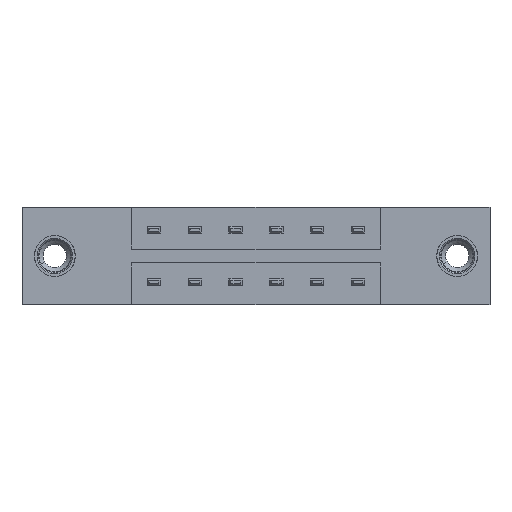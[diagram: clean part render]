
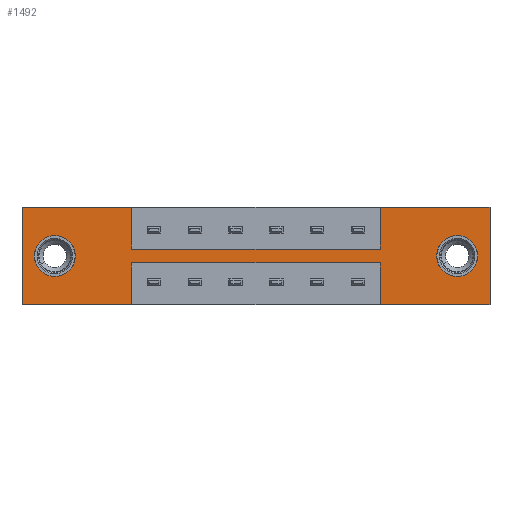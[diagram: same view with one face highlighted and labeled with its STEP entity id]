
A CAD part, front view. The second image highlights one B-rep face of the part: STEP entity #1492.
In plain terms, the highlighted planar face has unit normal (0, -1, 0).
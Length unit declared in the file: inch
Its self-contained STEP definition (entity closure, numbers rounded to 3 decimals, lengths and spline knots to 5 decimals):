
#13 = ORIENTED_EDGE ( 'NONE', *, *, #5651, .T. ) ;
#305 = ORIENTED_EDGE ( 'NONE', *, *, #8536, .F. ) ;
#362 = AXIS2_PLACEMENT_3D ( 'NONE', #4719, #4704, #4684 ) ;
#561 = VECTOR ( 'NONE', #1342, 39.37008 ) ;
#596 = DIRECTION ( 'NONE',  ( 0., 0., 1. ) ) ;
#611 = DIRECTION ( 'NONE',  ( 0., 1., 0. ) ) ;
#632 = CARTESIAN_POINT ( 'NONE',  ( 0.125, 0., -0.185 ) ) ;
#669 = ORIENTED_EDGE ( 'NONE', *, *, #1375, .T. ) ;
#816 = VERTEX_POINT ( 'NONE', #7714 ) ;
#878 = LINE ( 'NONE', #2511, #6748 ) ;
#913 = EDGE_CURVE ( 'NONE', #7745, #5572, #878, .T. ) ;
#1073 = VECTOR ( 'NONE', #7024, 39.37008 ) ;
#1323 = EDGE_CURVE ( 'NONE', #5572, #7181, #4646, .T. ) ;
#1342 = DIRECTION ( 'NONE',  ( 0., 0., 1. ) ) ;
#1375 = EDGE_CURVE ( 'NONE', #6483, #5742, #3723, .T. ) ;
#1381 = EDGE_LOOP ( 'NONE', ( #4957, #2207, #7634, #305, #5319, #8008, #8800, #1449, #4160, #9099, #5473, #8551 ) ) ;
#1449 = ORIENTED_EDGE ( 'NONE', *, *, #7810, .F. ) ;
#1492 = ADVANCED_FACE ( 'NONE', ( #7699, #2367, #5896 ), #2738, .T. ) ;
#1685 = CARTESIAN_POINT ( 'NONE',  ( 1.784, 0., 0. ) ) ;
#1892 = CARTESIAN_POINT ( 'NONE',  ( 1.3665, 0., -0.1585 ) ) ;
#1949 = VERTEX_POINT ( 'NONE', #8513 ) ;
#2194 = VERTEX_POINT ( 'NONE', #6733 ) ;
#2195 = LINE ( 'NONE', #5640, #9402 ) ;
#2207 = ORIENTED_EDGE ( 'NONE', *, *, #913, .F. ) ;
#2288 = VERTEX_POINT ( 'NONE', #5562 ) ;
#2299 = LINE ( 'NONE', #7814, #5845 ) ;
#2314 = LINE ( 'NONE', #1685, #7653 ) ;
#2346 = DIRECTION ( 'NONE',  ( -1., 0., 0. ) ) ;
#2367 = FACE_BOUND ( 'NONE', #9194, .T. ) ;
#2501 = VECTOR ( 'NONE', #6003, 39.37008 ) ;
#2511 = CARTESIAN_POINT ( 'NONE',  ( 0., 0., -0.37 ) ) ;
#2539 = LINE ( 'NONE', #6915, #6027 ) ;
#2600 = EDGE_CURVE ( 'NONE', #2288, #8261, #2843, .T. ) ;
#2736 = DIRECTION ( 'NONE',  ( 0., 0., -1. ) ) ;
#2738 = PLANE ( 'NONE',  #8091 ) ;
#2800 = CARTESIAN_POINT ( 'NONE',  ( 0.125, 0., -0.107 ) ) ;
#2802 = CARTESIAN_POINT ( 'NONE',  ( 0., 0., -0.37 ) ) ;
#2821 = LINE ( 'NONE', #5255, #8122 ) ;
#2832 = DIRECTION ( 'NONE',  ( 0., -1., 0. ) ) ;
#2843 = LINE ( 'NONE', #1892, #561 ) ;
#3033 = EDGE_CURVE ( 'NONE', #4695, #816, #2539, .T. ) ;
#3245 = DIRECTION ( 'NONE',  ( 0., 0., -1. ) ) ;
#3529 = CIRCLE ( 'NONE', #9371, 0.078 ) ;
#3587 = CARTESIAN_POINT ( 'NONE',  ( 1.659, 0., -0.185 ) ) ;
#3657 = VERTEX_POINT ( 'NONE', #8221 ) ;
#3663 = CARTESIAN_POINT ( 'NONE',  ( 0., 0., 0. ) ) ;
#3723 = CIRCLE ( 'NONE', #362, 0.078 ) ;
#3750 = ORIENTED_EDGE ( 'NONE', *, *, #4228, .T. ) ;
#3890 = AXIS2_PLACEMENT_3D ( 'NONE', #8607, #4503, #9289 ) ;
#3987 = CARTESIAN_POINT ( 'NONE',  ( 1.784, 0., -0.37 ) ) ;
#4000 = CIRCLE ( 'NONE', #3890, 0.078 ) ;
#4160 = ORIENTED_EDGE ( 'NONE', *, *, #6624, .F. ) ;
#4217 = CARTESIAN_POINT ( 'NONE',  ( 1.659, 0., -0.263 ) ) ;
#4228 = EDGE_CURVE ( 'NONE', #5742, #6483, #3529, .T. ) ;
#4321 = DIRECTION ( 'NONE',  ( 0., 0., -1. ) ) ;
#4322 = CARTESIAN_POINT ( 'NONE',  ( 0.4175, 0., -0.2115 ) ) ;
#4503 = DIRECTION ( 'NONE',  ( 0., 1., 0. ) ) ;
#4579 = DIRECTION ( 'NONE',  ( 0., 0., -1. ) ) ;
#4646 = LINE ( 'NONE', #6122, #2501 ) ;
#4684 = DIRECTION ( 'NONE',  ( 0., 0., 1. ) ) ;
#4695 = VERTEX_POINT ( 'NONE', #9009 ) ;
#4704 = DIRECTION ( 'NONE',  ( 0., 1., 0. ) ) ;
#4719 = CARTESIAN_POINT ( 'NONE',  ( 0.125, 0., -0.185 ) ) ;
#4920 = AXIS2_PLACEMENT_3D ( 'NONE', #3587, #8415, #4321 ) ;
#4957 = ORIENTED_EDGE ( 'NONE', *, *, #1323, .F. ) ;
#5255 = CARTESIAN_POINT ( 'NONE',  ( 0.4175, 0., -0.2115 ) ) ;
#5307 = CARTESIAN_POINT ( 'NONE',  ( 0., 0., 0. ) ) ;
#5319 = ORIENTED_EDGE ( 'NONE', *, *, #2600, .F. ) ;
#5473 = ORIENTED_EDGE ( 'NONE', *, *, #6842, .F. ) ;
#5562 = CARTESIAN_POINT ( 'NONE',  ( 1.3665, 0., -0.1585 ) ) ;
#5572 = VERTEX_POINT ( 'NONE', #8354 ) ;
#5640 = CARTESIAN_POINT ( 'NONE',  ( 0.4175, 0., -0.1585 ) ) ;
#5651 = EDGE_CURVE ( 'NONE', #6443, #3657, #7796, .T. ) ;
#5742 = VERTEX_POINT ( 'NONE', #8479 ) ;
#5754 = LINE ( 'NONE', #7459, #8986 ) ;
#5770 = CARTESIAN_POINT ( 'NONE',  ( 0.4175, 0., -0.1585 ) ) ;
#5845 = VECTOR ( 'NONE', #7117, 39.37008 ) ;
#5896 = FACE_OUTER_BOUND ( 'NONE', #1381, .T. ) ;
#6003 = DIRECTION ( 'NONE',  ( 0., 0., 1. ) ) ;
#6027 = VECTOR ( 'NONE', #6823, 39.37008 ) ;
#6078 = EDGE_LOOP ( 'NONE', ( #8168, #13 ) ) ;
#6122 = CARTESIAN_POINT ( 'NONE',  ( 1.3665, 0., -0.2115 ) ) ;
#6177 = LINE ( 'NONE', #3663, #6397 ) ;
#6312 = DIRECTION ( 'NONE',  ( 0., 0., -1. ) ) ;
#6318 = CARTESIAN_POINT ( 'NONE',  ( 0.4175, 0., -0.2115 ) ) ;
#6397 = VECTOR ( 'NONE', #9186, 39.37008 ) ;
#6443 = VERTEX_POINT ( 'NONE', #4217 ) ;
#6483 = VERTEX_POINT ( 'NONE', #2800 ) ;
#6516 = VERTEX_POINT ( 'NONE', #6318 ) ;
#6624 = EDGE_CURVE ( 'NONE', #816, #7606, #6177, .T. ) ;
#6733 = CARTESIAN_POINT ( 'NONE',  ( 0.4175, 0., 0. ) ) ;
#6748 = VECTOR ( 'NONE', #2346, 39.37008 ) ;
#6823 = DIRECTION ( 'NONE',  ( -1., 0., 0. ) ) ;
#6842 = EDGE_CURVE ( 'NONE', #6516, #4695, #2821, .T. ) ;
#6907 = CARTESIAN_POINT ( 'NONE',  ( 1.3665, 0., 0. ) ) ;
#6915 = CARTESIAN_POINT ( 'NONE',  ( 0., 0., -0.37 ) ) ;
#7024 = DIRECTION ( 'NONE',  ( -1., 0., 0. ) ) ;
#7117 = DIRECTION ( 'NONE',  ( 1., 0., 0. ) ) ;
#7181 = VERTEX_POINT ( 'NONE', #7523 ) ;
#7187 = EDGE_CURVE ( 'NONE', #2194, #1949, #2195, .T. ) ;
#7254 = DIRECTION ( 'NONE',  ( 1., 0., 0. ) ) ;
#7459 = CARTESIAN_POINT ( 'NONE',  ( 0., 0., 0. ) ) ;
#7523 = CARTESIAN_POINT ( 'NONE',  ( 1.3665, 0., -0.2115 ) ) ;
#7606 = VERTEX_POINT ( 'NONE', #5307 ) ;
#7634 = ORIENTED_EDGE ( 'NONE', *, *, #8826, .F. ) ;
#7653 = VECTOR ( 'NONE', #3245, 39.37008 ) ;
#7699 = FACE_BOUND ( 'NONE', #6078, .T. ) ;
#7714 = CARTESIAN_POINT ( 'NONE',  ( 0., 0., -0.37 ) ) ;
#7745 = VERTEX_POINT ( 'NONE', #3987 ) ;
#7796 = CIRCLE ( 'NONE', #4920, 0.078 ) ;
#7810 = EDGE_CURVE ( 'NONE', #7606, #2194, #5754, .T. ) ;
#7814 = CARTESIAN_POINT ( 'NONE',  ( 0., 0., 0. ) ) ;
#7861 = VECTOR ( 'NONE', #9201, 39.37008 ) ;
#8008 = ORIENTED_EDGE ( 'NONE', *, *, #8491, .F. ) ;
#8091 = AXIS2_PLACEMENT_3D ( 'NONE', #2802, #2832, #2736 ) ;
#8093 = LINE ( 'NONE', #5770, #7861 ) ;
#8122 = VECTOR ( 'NONE', #4579, 39.37008 ) ;
#8168 = ORIENTED_EDGE ( 'NONE', *, *, #8603, .T. ) ;
#8221 = CARTESIAN_POINT ( 'NONE',  ( 1.659, 0., -0.107 ) ) ;
#8261 = VERTEX_POINT ( 'NONE', #6907 ) ;
#8269 = VERTEX_POINT ( 'NONE', #8323 ) ;
#8323 = CARTESIAN_POINT ( 'NONE',  ( 1.784, 0., 0. ) ) ;
#8354 = CARTESIAN_POINT ( 'NONE',  ( 1.3665, 0., -0.37 ) ) ;
#8375 = EDGE_CURVE ( 'NONE', #7181, #6516, #8761, .T. ) ;
#8415 = DIRECTION ( 'NONE',  ( 0., 1., 0. ) ) ;
#8479 = CARTESIAN_POINT ( 'NONE',  ( 0.125, 0., -0.263 ) ) ;
#8491 = EDGE_CURVE ( 'NONE', #1949, #2288, #8093, .T. ) ;
#8513 = CARTESIAN_POINT ( 'NONE',  ( 0.4175, 0., -0.1585 ) ) ;
#8536 = EDGE_CURVE ( 'NONE', #8261, #8269, #2299, .T. ) ;
#8551 = ORIENTED_EDGE ( 'NONE', *, *, #8375, .F. ) ;
#8603 = EDGE_CURVE ( 'NONE', #3657, #6443, #4000, .T. ) ;
#8607 = CARTESIAN_POINT ( 'NONE',  ( 1.659, 0., -0.185 ) ) ;
#8761 = LINE ( 'NONE', #4322, #1073 ) ;
#8800 = ORIENTED_EDGE ( 'NONE', *, *, #7187, .F. ) ;
#8826 = EDGE_CURVE ( 'NONE', #8269, #7745, #2314, .T. ) ;
#8986 = VECTOR ( 'NONE', #7254, 39.37008 ) ;
#9009 = CARTESIAN_POINT ( 'NONE',  ( 0.4175, 0., -0.37 ) ) ;
#9099 = ORIENTED_EDGE ( 'NONE', *, *, #3033, .F. ) ;
#9186 = DIRECTION ( 'NONE',  ( 0., 0., 1. ) ) ;
#9194 = EDGE_LOOP ( 'NONE', ( #669, #3750 ) ) ;
#9201 = DIRECTION ( 'NONE',  ( 1., 0., 0. ) ) ;
#9289 = DIRECTION ( 'NONE',  ( 0., 0., -1. ) ) ;
#9371 = AXIS2_PLACEMENT_3D ( 'NONE', #632, #611, #596 ) ;
#9402 = VECTOR ( 'NONE', #6312, 39.37008 ) ;
